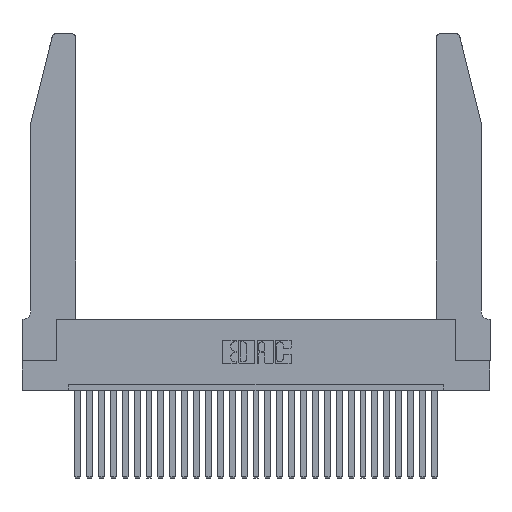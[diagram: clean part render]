
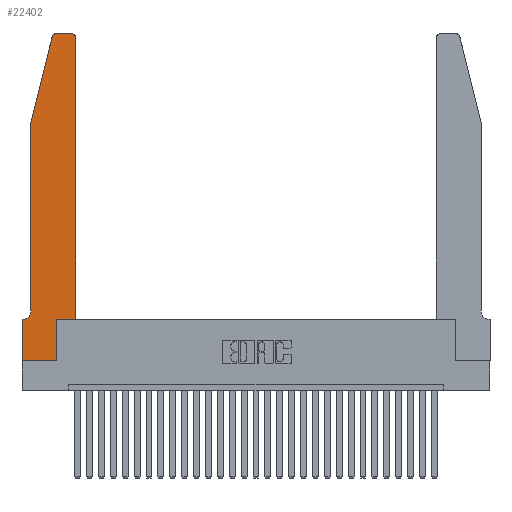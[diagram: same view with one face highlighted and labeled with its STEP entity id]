
A CAD part, top view. The second image highlights one B-rep face of the part: STEP entity #22402.
In plain terms, the highlighted planar face has unit normal (0, 0, 1).
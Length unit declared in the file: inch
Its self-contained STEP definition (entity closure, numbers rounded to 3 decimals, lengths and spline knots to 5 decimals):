
#302 = CARTESIAN_POINT ( 'NONE',  ( 0.2865, 0.35, 0.37 ) ) ;
#455 = EDGE_CURVE ( 'NONE', #8909, #7138, #1613, .T. ) ;
#1096 = LINE ( 'NONE', #4870, #20602 ) ;
#1613 = LINE ( 'NONE', #11443, #11899 ) ;
#1848 = VECTOR ( 'NONE', #9023, 39.37008 ) ;
#2285 = CARTESIAN_POINT ( 'NONE',  ( 0.0755, 2., 0.37 ) ) ;
#2493 = DIRECTION ( 'NONE',  ( 0., -1., 0. ) ) ;
#2715 = DIRECTION ( 'NONE',  ( 1., 0., 0. ) ) ;
#2717 = DIRECTION ( 'NONE',  ( 0., 0., -1. ) ) ;
#2760 = ORIENTED_EDGE ( 'NONE', *, *, #6442, .T. ) ;
#4371 = ORIENTED_EDGE ( 'NONE', *, *, #19651, .T. ) ;
#4564 = CARTESIAN_POINT ( 'NONE',  ( 0.0755, 0.42, 0.37 ) ) ;
#4599 = EDGE_CURVE ( 'NONE', #24689, #19361, #6574, .T. ) ;
#4870 = CARTESIAN_POINT ( 'NONE',  ( 0.4505, 0.35, 0.37 ) ) ;
#4894 = ORIENTED_EDGE ( 'NONE', *, *, #4599, .T. ) ;
#5000 = DIRECTION ( 'NONE',  ( -1., 0., 0. ) ) ;
#5283 = VERTEX_POINT ( 'NONE', #27171 ) ;
#5383 = EDGE_LOOP ( 'NONE', ( #2760, #4371, #17296, #28122, #8143, #24431, #4894, #16472, #17223, #17024, #16028, #8445 ) ) ;
#5705 = DIRECTION ( 'NONE',  ( 0., 0., 1. ) ) ;
#5719 = DIRECTION ( 'NONE',  ( 0., 1., 0. ) ) ;
#5781 = CIRCLE ( 'NONE', #27266, 0.07 ) ;
#6065 = VECTOR ( 'NONE', #23451, 39.37008 ) ;
#6302 = CARTESIAN_POINT ( 'NONE',  ( 0., 0., 0.37 ) ) ;
#6309 = CARTESIAN_POINT ( 'NONE',  ( 0.25487, 2.72718, 0.37 ) ) ;
#6324 = VERTEX_POINT ( 'NONE', #17448 ) ;
#6442 = EDGE_CURVE ( 'NONE', #21536, #24987, #26335, .T. ) ;
#6574 = LINE ( 'NONE', #13227, #18242 ) ;
#6703 = DIRECTION ( 'NONE',  ( -0.239, -0.971, 0. ) ) ;
#7138 = VERTEX_POINT ( 'NONE', #9072 ) ;
#7236 = DIRECTION ( 'NONE',  ( 0., 1., 0. ) ) ;
#7490 = LINE ( 'NONE', #12334, #6065 ) ;
#8143 = ORIENTED_EDGE ( 'NONE', *, *, #15666, .T. ) ;
#8445 = ORIENTED_EDGE ( 'NONE', *, *, #16135, .T. ) ;
#8591 = FACE_OUTER_BOUND ( 'NONE', #5383, .T. ) ;
#8909 = VERTEX_POINT ( 'NONE', #6309 ) ;
#9001 = CARTESIAN_POINT ( 'NONE',  ( 0.4505, 2.72, 0.37 ) ) ;
#9023 = DIRECTION ( 'NONE',  ( -1., 0., 0. ) ) ;
#9072 = CARTESIAN_POINT ( 'NONE',  ( 0.0755, 2., 0.37 ) ) ;
#10068 = CARTESIAN_POINT ( 'NONE',  ( 0.4505, 0.35, 0.37 ) ) ;
#10251 = DIRECTION ( 'NONE',  ( -1., 0., 0. ) ) ;
#10305 = EDGE_CURVE ( 'NONE', #7138, #13800, #20534, .T. ) ;
#10396 = VERTEX_POINT ( 'NONE', #19078 ) ;
#11292 = VERTEX_POINT ( 'NONE', #9001 ) ;
#11443 = CARTESIAN_POINT ( 'NONE',  ( 0.0755, 2., 0.37 ) ) ;
#11899 = VECTOR ( 'NONE', #6703, 39.37008 ) ;
#12273 = EDGE_CURVE ( 'NONE', #15225, #11292, #12986, .T. ) ;
#12334 = CARTESIAN_POINT ( 'NONE',  ( 0., 0., 0.37 ) ) ;
#12799 = CARTESIAN_POINT ( 'NONE',  ( 0.4205, 2.72, 0.37 ) ) ;
#12986 = LINE ( 'NONE', #10068, #22918 ) ;
#12996 = CARTESIAN_POINT ( 'NONE',  ( 0., 0.35, 0.37 ) ) ;
#13227 = CARTESIAN_POINT ( 'NONE',  ( 0., 0., 0.37 ) ) ;
#13800 = VERTEX_POINT ( 'NONE', #4564 ) ;
#13975 = EDGE_CURVE ( 'NONE', #10396, #5283, #20661, .T. ) ;
#14112 = CARTESIAN_POINT ( 'NONE',  ( 0.4505, 0.35, 0.37 ) ) ;
#14118 = PLANE ( 'NONE',  #28519 ) ;
#14715 = EDGE_CURVE ( 'NONE', #6324, #24689, #25284, .T. ) ;
#15225 = VERTEX_POINT ( 'NONE', #14112 ) ;
#15666 = EDGE_CURVE ( 'NONE', #13800, #6324, #5781, .T. ) ;
#16028 = ORIENTED_EDGE ( 'NONE', *, *, #12273, .T. ) ;
#16085 = CARTESIAN_POINT ( 'NONE',  ( 0., 0.35, 0.37 ) ) ;
#16135 = EDGE_CURVE ( 'NONE', #11292, #21536, #25958, .T. ) ;
#16472 = ORIENTED_EDGE ( 'NONE', *, *, #17235, .T. ) ;
#16645 = CARTESIAN_POINT ( 'NONE',  ( 0.284, 2.75, 0.37 ) ) ;
#16972 = CARTESIAN_POINT ( 'NONE',  ( 0.284, 2.72, 0.37 ) ) ;
#17024 = ORIENTED_EDGE ( 'NONE', *, *, #17165, .T. ) ;
#17165 = EDGE_CURVE ( 'NONE', #5283, #15225, #1096, .T. ) ;
#17223 = ORIENTED_EDGE ( 'NONE', *, *, #13975, .T. ) ;
#17235 = EDGE_CURVE ( 'NONE', #19361, #10396, #7490, .T. ) ;
#17296 = ORIENTED_EDGE ( 'NONE', *, *, #455, .T. ) ;
#17448 = CARTESIAN_POINT ( 'NONE',  ( 0.0055, 0.35, 0.37 ) ) ;
#17903 = CARTESIAN_POINT ( 'NONE',  ( 0.4205, 2.75, 0.37 ) ) ;
#18242 = VECTOR ( 'NONE', #20039, 39.37008 ) ;
#18498 = VECTOR ( 'NONE', #10251, 39.37008 ) ;
#19078 = CARTESIAN_POINT ( 'NONE',  ( 0.2865, 0., 0.37 ) ) ;
#19361 = VERTEX_POINT ( 'NONE', #6302 ) ;
#19651 = EDGE_CURVE ( 'NONE', #24987, #8909, #29309, .T. ) ;
#19932 = VECTOR ( 'NONE', #7236, 39.37008 ) ;
#20039 = DIRECTION ( 'NONE',  ( 0., -1., 0. ) ) ;
#20534 = LINE ( 'NONE', #2285, #25863 ) ;
#20592 = CARTESIAN_POINT ( 'NONE',  ( 0.0055, 0.42, 0.37 ) ) ;
#20602 = VECTOR ( 'NONE', #27983, 39.37008 ) ;
#20661 = LINE ( 'NONE', #302, #19932 ) ;
#21383 = CARTESIAN_POINT ( 'NONE',  ( 0.0755, 0.35, 0.37 ) ) ;
#21536 = VERTEX_POINT ( 'NONE', #17903 ) ;
#21723 = DIRECTION ( 'NONE',  ( 0., 0., 1. ) ) ;
#22402 = ADVANCED_FACE ( 'NONE', ( #8591 ), #14118, .T. ) ;
#22619 = CARTESIAN_POINT ( 'NONE',  ( 0.2605, 2.75, 0.37 ) ) ;
#22803 = AXIS2_PLACEMENT_3D ( 'NONE', #16972, #5705, #28978 ) ;
#22918 = VECTOR ( 'NONE', #5719, 39.37008 ) ;
#23451 = DIRECTION ( 'NONE',  ( 1., 0., 0. ) ) ;
#24431 = ORIENTED_EDGE ( 'NONE', *, *, #14715, .T. ) ;
#24689 = VERTEX_POINT ( 'NONE', #12996 ) ;
#24987 = VERTEX_POINT ( 'NONE', #16645 ) ;
#25134 = DIRECTION ( 'NONE',  ( 0., 0., 1. ) ) ;
#25284 = LINE ( 'NONE', #21383, #18498 ) ;
#25863 = VECTOR ( 'NONE', #2493, 39.37008 ) ;
#25958 = CIRCLE ( 'NONE', #28791, 0.03 ) ;
#26335 = LINE ( 'NONE', #22619, #1848 ) ;
#26368 = DIRECTION ( 'NONE',  ( 1., 0., 0. ) ) ;
#27171 = CARTESIAN_POINT ( 'NONE',  ( 0.2865, 0.35, 0.37 ) ) ;
#27266 = AXIS2_PLACEMENT_3D ( 'NONE', #20592, #2717, #5000 ) ;
#27983 = DIRECTION ( 'NONE',  ( 1., 0., 0. ) ) ;
#28122 = ORIENTED_EDGE ( 'NONE', *, *, #10305, .T. ) ;
#28519 = AXIS2_PLACEMENT_3D ( 'NONE', #16085, #25134, #2715 ) ;
#28791 = AXIS2_PLACEMENT_3D ( 'NONE', #12799, #21723, #26368 ) ;
#28978 = DIRECTION ( 'NONE',  ( 1., 0., 0. ) ) ;
#29309 = CIRCLE ( 'NONE', #22803, 0.03 ) ;
